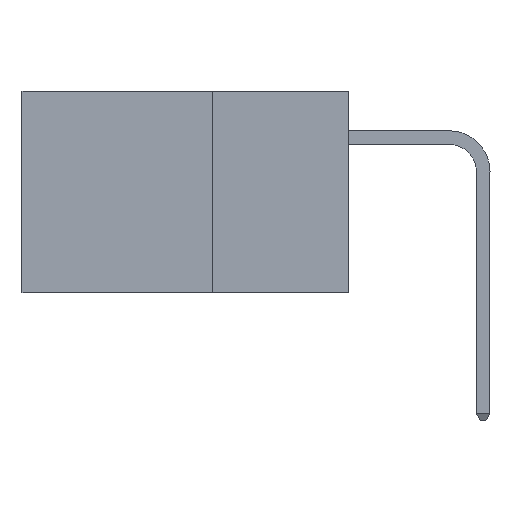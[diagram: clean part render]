
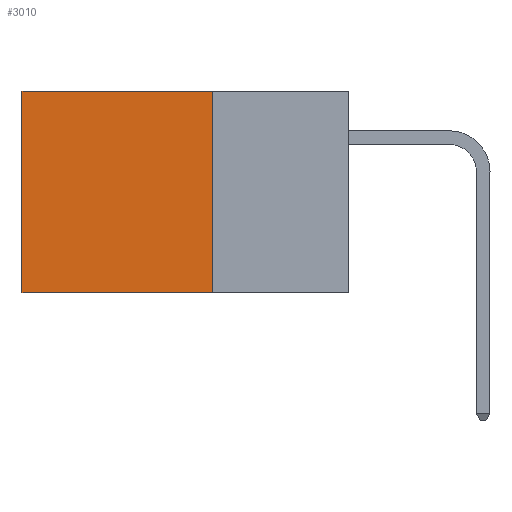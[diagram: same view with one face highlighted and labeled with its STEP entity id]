
A CAD part, left-side view. The second image highlights one B-rep face of the part: STEP entity #3010.
In plain terms, the highlighted planar face has unit normal (-1, 0, 0).
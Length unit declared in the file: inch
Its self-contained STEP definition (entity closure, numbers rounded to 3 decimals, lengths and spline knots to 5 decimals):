
#335 = CARTESIAN_POINT ( 'NONE',  ( 0.2875, 0.6, 0. ) ) ;
#526 = DIRECTION ( 'NONE',  ( 0., 0., -1. ) ) ;
#639 = ORIENTED_EDGE ( 'NONE', *, *, #4676, .T. ) ;
#1493 = EDGE_CURVE ( 'NONE', #16764, #16146, #3592, .T. ) ;
#1941 = VERTEX_POINT ( 'NONE', #3353 ) ;
#1983 = EDGE_CURVE ( 'NONE', #18058, #16146, #11783, .T. ) ;
#2123 = CARTESIAN_POINT ( 'NONE',  ( 0.2875, 0.25, -0.37 ) ) ;
#3010 = ADVANCED_FACE ( 'NONE', ( #12996 ), #8163, .F. ) ;
#3200 = CARTESIAN_POINT ( 'NONE',  ( 0.2875, 0.25, 0. ) ) ;
#3335 = ORIENTED_EDGE ( 'NONE', *, *, #1983, .F. ) ;
#3353 = CARTESIAN_POINT ( 'NONE',  ( 0.2875, 0.25, 0. ) ) ;
#3592 = LINE ( 'NONE', #13672, #20375 ) ;
#4393 = AXIS2_PLACEMENT_3D ( 'NONE', #3200, #19487, #9836 ) ;
#4676 = EDGE_CURVE ( 'NONE', #1941, #16764, #10648, .T. ) ;
#5241 = VECTOR ( 'NONE', #18720, 39.37008 ) ;
#6653 = DIRECTION ( 'NONE',  ( 0., 1., 0. ) ) ;
#7109 = VECTOR ( 'NONE', #13687, 39.37008 ) ;
#7599 = ORIENTED_EDGE ( 'NONE', *, *, #20170, .F. ) ;
#8163 = PLANE ( 'NONE',  #4393 ) ;
#8223 = EDGE_LOOP ( 'NONE', ( #19731, #3335, #7599, #639 ) ) ;
#9836 = DIRECTION ( 'NONE',  ( 0., 0., -1. ) ) ;
#10648 = LINE ( 'NONE', #20334, #5241 ) ;
#11274 = VECTOR ( 'NONE', #6653, 39.37008 ) ;
#11783 = LINE ( 'NONE', #13229, #11274 ) ;
#12996 = FACE_OUTER_BOUND ( 'NONE', #8223, .T. ) ;
#13229 = CARTESIAN_POINT ( 'NONE',  ( 0.2875, 0.25, -0.37 ) ) ;
#13672 = CARTESIAN_POINT ( 'NONE',  ( 0.2875, 0.6, 0. ) ) ;
#13687 = DIRECTION ( 'NONE',  ( 0., 0., -1. ) ) ;
#16146 = VERTEX_POINT ( 'NONE', #16836 ) ;
#16764 = VERTEX_POINT ( 'NONE', #335 ) ;
#16836 = CARTESIAN_POINT ( 'NONE',  ( 0.2875, 0.6, -0.37 ) ) ;
#18058 = VERTEX_POINT ( 'NONE', #2123 ) ;
#18720 = DIRECTION ( 'NONE',  ( 0., 1., 0. ) ) ;
#19487 = DIRECTION ( 'NONE',  ( 1., 0., 0. ) ) ;
#19731 = ORIENTED_EDGE ( 'NONE', *, *, #1493, .T. ) ;
#20044 = LINE ( 'NONE', #20086, #7109 ) ;
#20086 = CARTESIAN_POINT ( 'NONE',  ( 0.2875, 0.25, 0. ) ) ;
#20170 = EDGE_CURVE ( 'NONE', #1941, #18058, #20044, .T. ) ;
#20334 = CARTESIAN_POINT ( 'NONE',  ( 0.2875, 0.25, 0. ) ) ;
#20375 = VECTOR ( 'NONE', #526, 39.37008 ) ;
